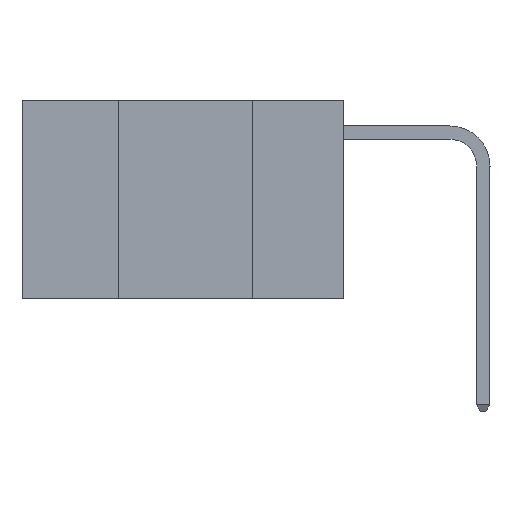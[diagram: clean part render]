
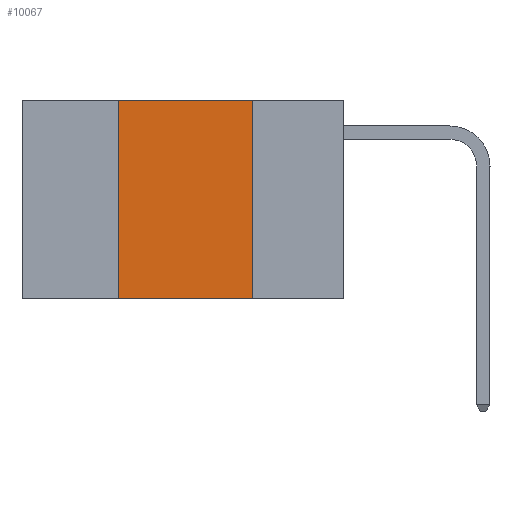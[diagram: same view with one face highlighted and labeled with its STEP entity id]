
A CAD part, left-side view. The second image highlights one B-rep face of the part: STEP entity #10067.
In plain terms, the highlighted planar face has unit normal (-1, 0, 0).
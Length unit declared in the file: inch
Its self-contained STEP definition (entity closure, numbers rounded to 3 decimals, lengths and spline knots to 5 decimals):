
#339 = CARTESIAN_POINT ( 'NONE',  ( 0., 0.42, -0.37 ) ) ;
#340 = CARTESIAN_POINT ( 'NONE',  ( 0., 0.42, 0. ) ) ;
#963 = CARTESIAN_POINT ( 'NONE',  ( 0., 0.6, 0. ) ) ;
#1313 = VECTOR ( 'NONE', #9323, 39.37008 ) ;
#1525 = CARTESIAN_POINT ( 'NONE',  ( 0., 0.42, 0. ) ) ;
#1574 = VERTEX_POINT ( 'NONE', #6111 ) ;
#1648 = LINE ( 'NONE', #963, #1313 ) ;
#2348 = EDGE_CURVE ( 'NONE', #1574, #11578, #3682, .T. ) ;
#3116 = DIRECTION ( 'NONE',  ( 0., -1., 0. ) ) ;
#3361 = VECTOR ( 'NONE', #6840, 39.37008 ) ;
#3439 = PLANE ( 'NONE',  #7037 ) ;
#3517 = CARTESIAN_POINT ( 'NONE',  ( 0., 0.17, -0.37 ) ) ;
#3526 = FACE_OUTER_BOUND ( 'NONE', #7470, .T. ) ;
#3682 = LINE ( 'NONE', #5755, #3361 ) ;
#3822 = ORIENTED_EDGE ( 'NONE', *, *, #2348, .F. ) ;
#4020 = EDGE_CURVE ( 'NONE', #7881, #11578, #11406, .T. ) ;
#4147 = ORIENTED_EDGE ( 'NONE', *, *, #12442, .F. ) ;
#4472 = DIRECTION ( 'NONE',  ( 1., 0., 0. ) ) ;
#5507 = VERTEX_POINT ( 'NONE', #1525 ) ;
#5755 = CARTESIAN_POINT ( 'NONE',  ( 0., 0.17, 0. ) ) ;
#6111 = CARTESIAN_POINT ( 'NONE',  ( 0., 0.17, 0. ) ) ;
#6233 = CARTESIAN_POINT ( 'NONE',  ( 0., 0.6, -0.37 ) ) ;
#6840 = DIRECTION ( 'NONE',  ( 0., 0., -1. ) ) ;
#6968 = ORIENTED_EDGE ( 'NONE', *, *, #10932, .F. ) ;
#7037 = AXIS2_PLACEMENT_3D ( 'NONE', #9646, #4472, #11655 ) ;
#7288 = ORIENTED_EDGE ( 'NONE', *, *, #4020, .T. ) ;
#7470 = EDGE_LOOP ( 'NONE', ( #3822, #4147, #6968, #7288 ) ) ;
#7881 = VERTEX_POINT ( 'NONE', #339 ) ;
#8390 = VECTOR ( 'NONE', #8718, 39.37008 ) ;
#8708 = LINE ( 'NONE', #340, #8390 ) ;
#8718 = DIRECTION ( 'NONE',  ( 0., 0., 1. ) ) ;
#9323 = DIRECTION ( 'NONE',  ( 0., -1., 0. ) ) ;
#9646 = CARTESIAN_POINT ( 'NONE',  ( 0., 0.6, 0. ) ) ;
#10067 = ADVANCED_FACE ( 'NONE', ( #3526 ), #3439, .F. ) ;
#10742 = VECTOR ( 'NONE', #3116, 39.37008 ) ;
#10932 = EDGE_CURVE ( 'NONE', #7881, #5507, #8708, .T. ) ;
#11406 = LINE ( 'NONE', #6233, #10742 ) ;
#11578 = VERTEX_POINT ( 'NONE', #3517 ) ;
#11655 = DIRECTION ( 'NONE',  ( 0., 0., -1. ) ) ;
#12442 = EDGE_CURVE ( 'NONE', #5507, #1574, #1648, .T. ) ;
